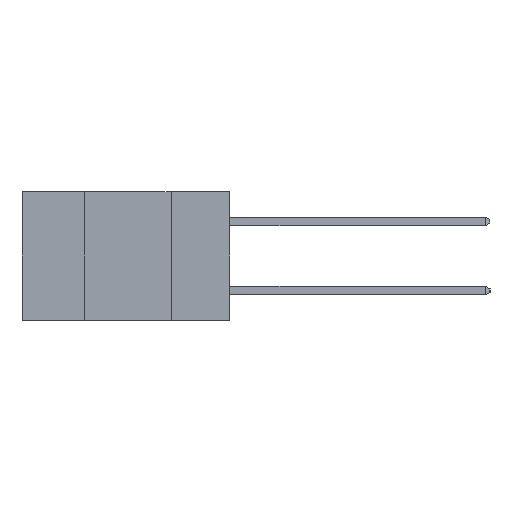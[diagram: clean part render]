
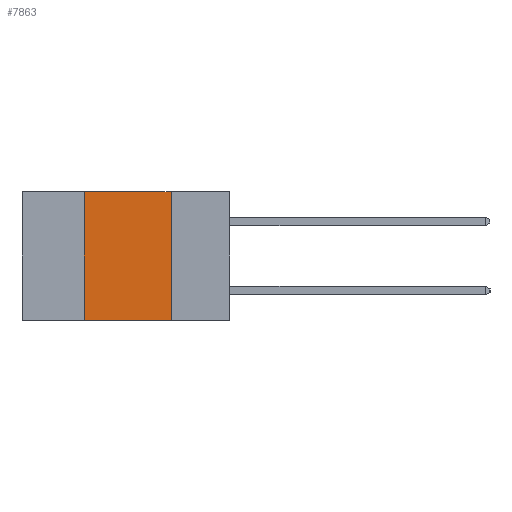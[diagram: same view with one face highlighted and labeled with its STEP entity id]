
A CAD part, left-side view. The second image highlights one B-rep face of the part: STEP entity #7863.
In plain terms, the highlighted planar face has unit normal (-1, 0, 0).
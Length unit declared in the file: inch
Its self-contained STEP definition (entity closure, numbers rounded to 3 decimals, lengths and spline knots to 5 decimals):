
#1088 = CARTESIAN_POINT ( 'NONE',  ( 0., 0.42, 0. ) ) ;
#1190 = VERTEX_POINT ( 'NONE', #7318 ) ;
#1329 = CARTESIAN_POINT ( 'NONE',  ( 0., 0.6, 0. ) ) ;
#1645 = CARTESIAN_POINT ( 'NONE',  ( 0., 0.42, -0.37 ) ) ;
#1840 = VERTEX_POINT ( 'NONE', #4295 ) ;
#1901 = DIRECTION ( 'NONE',  ( 0., 0., 1. ) ) ;
#2233 = EDGE_CURVE ( 'NONE', #1840, #5293, #6144, .T. ) ;
#2798 = AXIS2_PLACEMENT_3D ( 'NONE', #8120, #3744, #8815 ) ;
#2848 = EDGE_CURVE ( 'NONE', #7399, #1190, #8616, .T. ) ;
#2883 = DIRECTION ( 'NONE',  ( 0., -1., 0. ) ) ;
#3289 = ORIENTED_EDGE ( 'NONE', *, *, #5510, .T. ) ;
#3301 = LINE ( 'NONE', #7313, #3541 ) ;
#3371 = EDGE_LOOP ( 'NONE', ( #6510, #6471, #9005, #3289 ) ) ;
#3541 = VECTOR ( 'NONE', #2883, 39.37008 ) ;
#3744 = DIRECTION ( 'NONE',  ( 1., 0., 0. ) ) ;
#3780 = CARTESIAN_POINT ( 'NONE',  ( 0., 0.17, 0. ) ) ;
#4295 = CARTESIAN_POINT ( 'NONE',  ( 0., 0.42, -0.37 ) ) ;
#5293 = VERTEX_POINT ( 'NONE', #1088 ) ;
#5510 = EDGE_CURVE ( 'NONE', #1840, #1190, #3301, .T. ) ;
#5907 = VECTOR ( 'NONE', #1901, 39.37008 ) ;
#6098 = FACE_OUTER_BOUND ( 'NONE', #3371, .T. ) ;
#6144 = LINE ( 'NONE', #1645, #5907 ) ;
#6471 = ORIENTED_EDGE ( 'NONE', *, *, #8438, .F. ) ;
#6510 = ORIENTED_EDGE ( 'NONE', *, *, #2848, .F. ) ;
#6703 = VECTOR ( 'NONE', #6899, 39.37008 ) ;
#6899 = DIRECTION ( 'NONE',  ( 0., 0., -1. ) ) ;
#7158 = CARTESIAN_POINT ( 'NONE',  ( 0., 0.17, -0.37 ) ) ;
#7285 = DIRECTION ( 'NONE',  ( 0., -1., 0. ) ) ;
#7313 = CARTESIAN_POINT ( 'NONE',  ( 0., 0.6, -0.37 ) ) ;
#7318 = CARTESIAN_POINT ( 'NONE',  ( 0., 0.17, -0.37 ) ) ;
#7350 = LINE ( 'NONE', #1329, #7797 ) ;
#7399 = VERTEX_POINT ( 'NONE', #3780 ) ;
#7797 = VECTOR ( 'NONE', #7285, 39.37008 ) ;
#7863 = ADVANCED_FACE ( 'NONE', ( #6098 ), #8095, .F. ) ;
#8095 = PLANE ( 'NONE',  #2798 ) ;
#8120 = CARTESIAN_POINT ( 'NONE',  ( 0., 0.6, 0. ) ) ;
#8438 = EDGE_CURVE ( 'NONE', #5293, #7399, #7350, .T. ) ;
#8616 = LINE ( 'NONE', #7158, #6703 ) ;
#8815 = DIRECTION ( 'NONE',  ( 0., 0., -1. ) ) ;
#9005 = ORIENTED_EDGE ( 'NONE', *, *, #2233, .F. ) ;
